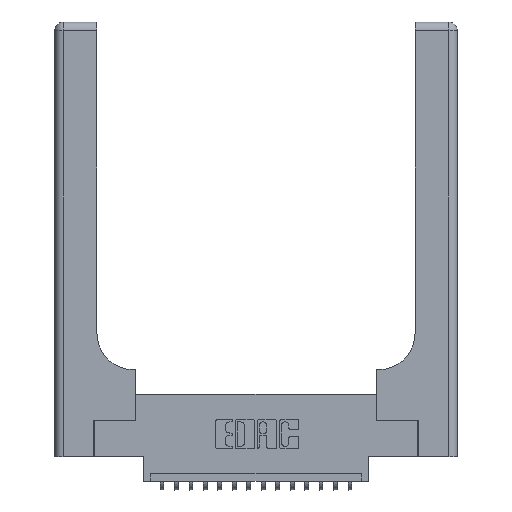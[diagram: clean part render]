
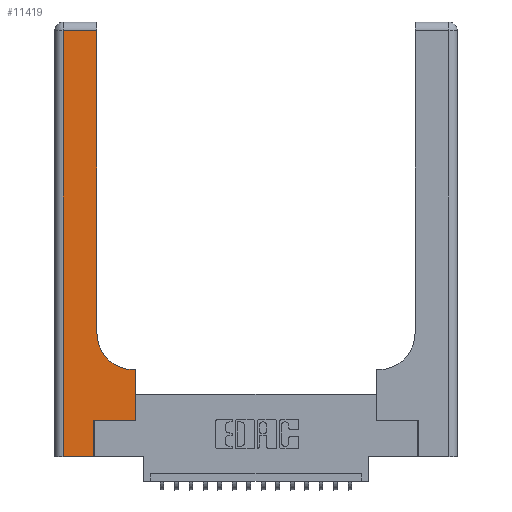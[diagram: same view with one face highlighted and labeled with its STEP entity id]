
A CAD part, top view. The second image highlights one B-rep face of the part: STEP entity #11419.
In plain terms, the highlighted planar face has unit normal (0, 0, 1).
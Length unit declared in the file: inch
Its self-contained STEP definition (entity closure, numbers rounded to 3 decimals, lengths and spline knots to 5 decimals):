
#23 = CARTESIAN_POINT ( 'NONE',  ( 0.269, 0.25, 0.37 ) ) ;
#75 = CARTESIAN_POINT ( 'NONE',  ( 0.06, 3., 0.37 ) ) ;
#106 = ORIENTED_EDGE ( 'NONE', *, *, #7964, .T. ) ;
#1189 = VERTEX_POINT ( 'NONE', #9747 ) ;
#1199 = AXIS2_PLACEMENT_3D ( 'NONE', #18516, #6689, #9423 ) ;
#1472 = ORIENTED_EDGE ( 'NONE', *, *, #12997, .T. ) ;
#1783 = LINE ( 'NONE', #13458, #12347 ) ;
#1796 = ORIENTED_EDGE ( 'NONE', *, *, #7412, .T. ) ;
#2326 = EDGE_CURVE ( 'NONE', #10774, #18113, #13433, .T. ) ;
#2374 = LINE ( 'NONE', #19119, #2622 ) ;
#2622 = VECTOR ( 'NONE', #17838, 39.37008 ) ;
#3831 = DIRECTION ( 'NONE',  ( -1., 0., 0. ) ) ;
#4382 = LINE ( 'NONE', #9695, #16242 ) ;
#4804 = FACE_OUTER_BOUND ( 'NONE', #5573, .T. ) ;
#4933 = CARTESIAN_POINT ( 'NONE',  ( 0.2915, 2.94, 0.37 ) ) ;
#5573 = EDGE_LOOP ( 'NONE', ( #1796, #6149, #11141, #14115, #6866, #8944, #11442, #1472, #106 ) ) ;
#5584 = CARTESIAN_POINT ( 'NONE',  ( 0.06, 2.94, 0.37 ) ) ;
#5944 = DIRECTION ( 'NONE',  ( 1., 0., 0. ) ) ;
#5998 = CARTESIAN_POINT ( 'NONE',  ( 0.5415, 0.85, 0.37 ) ) ;
#6118 = DIRECTION ( 'NONE',  ( 0., 1., 0. ) ) ;
#6132 = DIRECTION ( 'NONE',  ( 0., 0., -1. ) ) ;
#6149 = ORIENTED_EDGE ( 'NONE', *, *, #17658, .T. ) ;
#6485 = LINE ( 'NONE', #8538, #18115 ) ;
#6689 = DIRECTION ( 'NONE',  ( 0., 0., -1. ) ) ;
#6810 = VERTEX_POINT ( 'NONE', #15889 ) ;
#6866 = ORIENTED_EDGE ( 'NONE', *, *, #15379, .T. ) ;
#6879 = VERTEX_POINT ( 'NONE', #16710 ) ;
#7412 = EDGE_CURVE ( 'NONE', #1189, #19444, #2374, .T. ) ;
#7647 = DIRECTION ( 'NONE',  ( 1., 0., 0. ) ) ;
#7648 = AXIS2_PLACEMENT_3D ( 'NONE', #5998, #6132, #7647 ) ;
#7964 = EDGE_CURVE ( 'NONE', #6879, #1189, #18742, .T. ) ;
#8538 = CARTESIAN_POINT ( 'NONE',  ( 0., 2.94, 0.37 ) ) ;
#8944 = ORIENTED_EDGE ( 'NONE', *, *, #2326, .T. ) ;
#9194 = CARTESIAN_POINT ( 'NONE',  ( 0.269, 0.25, 0.37 ) ) ;
#9423 = DIRECTION ( 'NONE',  ( -1., 0., 0. ) ) ;
#9508 = EDGE_CURVE ( 'NONE', #17136, #6810, #1783, .T. ) ;
#9695 = CARTESIAN_POINT ( 'NONE',  ( 0.269, 0., 0.37 ) ) ;
#9747 = CARTESIAN_POINT ( 'NONE',  ( 0.2915, 0.85, 0.37 ) ) ;
#10774 = VERTEX_POINT ( 'NONE', #9194 ) ;
#11141 = ORIENTED_EDGE ( 'NONE', *, *, #15658, .T. ) ;
#11162 = DIRECTION ( 'NONE',  ( -1., 0., 0. ) ) ;
#11419 = ADVANCED_FACE ( 'NONE', ( #4804 ), #12739, .F. ) ;
#11442 = ORIENTED_EDGE ( 'NONE', *, *, #19344, .T. ) ;
#12347 = VECTOR ( 'NONE', #5944, 39.37008 ) ;
#12486 = VECTOR ( 'NONE', #18249, 39.37008 ) ;
#12739 = PLANE ( 'NONE',  #1199 ) ;
#12907 = LINE ( 'NONE', #75, #15770 ) ;
#12933 = DIRECTION ( 'NONE',  ( 0., 1., 0. ) ) ;
#12953 = CARTESIAN_POINT ( 'NONE',  ( 0.2915, 0.6, 0.37 ) ) ;
#12997 = EDGE_CURVE ( 'NONE', #16086, #6879, #17773, .T. ) ;
#13433 = LINE ( 'NONE', #23, #12486 ) ;
#13458 = CARTESIAN_POINT ( 'NONE',  ( 0., 0., 0.37 ) ) ;
#13728 = DIRECTION ( 'NONE',  ( 0., -1., 0. ) ) ;
#13762 = VECTOR ( 'NONE', #11162, 39.37008 ) ;
#14115 = ORIENTED_EDGE ( 'NONE', *, *, #9508, .T. ) ;
#14664 = CARTESIAN_POINT ( 'NONE',  ( 0.06, 0., 0.37 ) ) ;
#15379 = EDGE_CURVE ( 'NONE', #6810, #10774, #4382, .T. ) ;
#15658 = EDGE_CURVE ( 'NONE', #19068, #17136, #12907, .T. ) ;
#15770 = VECTOR ( 'NONE', #13728, 39.37008 ) ;
#15889 = CARTESIAN_POINT ( 'NONE',  ( 0.269, 0., 0.37 ) ) ;
#16086 = VERTEX_POINT ( 'NONE', #19359 ) ;
#16242 = VECTOR ( 'NONE', #12933, 39.37008 ) ;
#16710 = CARTESIAN_POINT ( 'NONE',  ( 0.5415, 0.6, 0.37 ) ) ;
#17136 = VERTEX_POINT ( 'NONE', #14664 ) ;
#17658 = EDGE_CURVE ( 'NONE', #19444, #19068, #6485, .T. ) ;
#17773 = LINE ( 'NONE', #12953, #13762 ) ;
#17838 = DIRECTION ( 'NONE',  ( 0., 1., 0. ) ) ;
#18113 = VERTEX_POINT ( 'NONE', #18947 ) ;
#18115 = VECTOR ( 'NONE', #3831, 39.37008 ) ;
#18249 = DIRECTION ( 'NONE',  ( 1., 0., 0. ) ) ;
#18297 = VECTOR ( 'NONE', #6118, 39.37008 ) ;
#18516 = CARTESIAN_POINT ( 'NONE',  ( 0., 3., 0.37 ) ) ;
#18742 = CIRCLE ( 'NONE', #7648, 0.25 ) ;
#18947 = CARTESIAN_POINT ( 'NONE',  ( 0.5585, 0.25, 0.37 ) ) ;
#19068 = VERTEX_POINT ( 'NONE', #5584 ) ;
#19119 = CARTESIAN_POINT ( 'NONE',  ( 0.2915, 3., 0.37 ) ) ;
#19344 = EDGE_CURVE ( 'NONE', #18113, #16086, #19477, .T. ) ;
#19359 = CARTESIAN_POINT ( 'NONE',  ( 0.5585, 0.6, 0.37 ) ) ;
#19444 = VERTEX_POINT ( 'NONE', #4933 ) ;
#19477 = LINE ( 'NONE', #19713, #18297 ) ;
#19713 = CARTESIAN_POINT ( 'NONE',  ( 0.5585, 0.25, 0.37 ) ) ;
